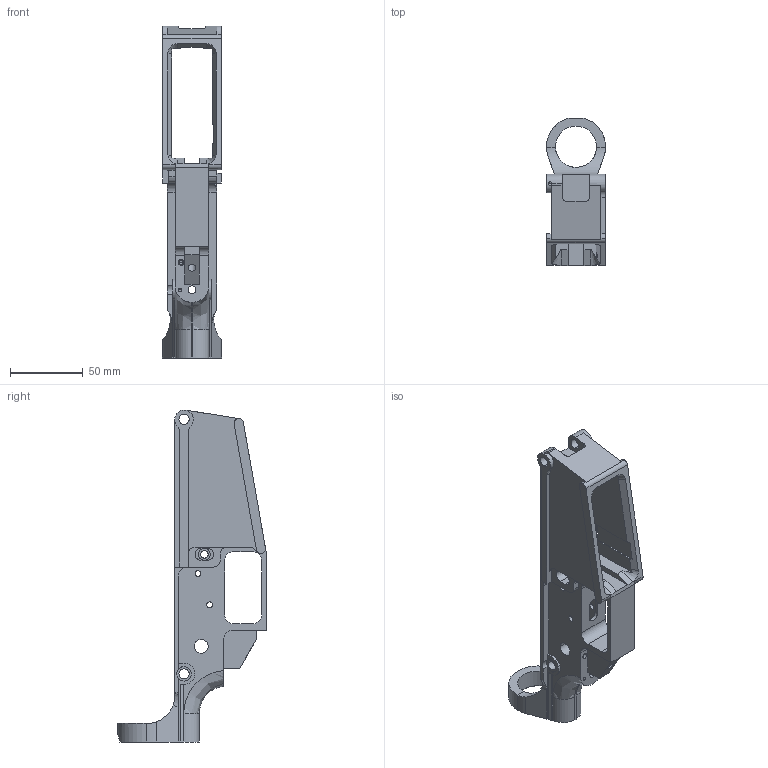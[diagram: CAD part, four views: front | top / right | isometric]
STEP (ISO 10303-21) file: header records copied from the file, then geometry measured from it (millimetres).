
FILE_DESCRIPTION (( 'STEP AP214' ), '1' );
FILE_NAME ('LR308 LOWER.STEP', '2016-04-23T05:09:30', ( '' ), ( '' ), 'SwSTEP 2.0', 'SolidWorks 2013', '' );
FILE_SCHEMA (( 'AUTOMOTIVE_DESIGN' ));
Length unit declared in the file: inch
Products named in the file (1): LR308 LOWER
Bounding box: 40.51 x 101.6 x 227.84 mm (x, y, z)
Volume: 130329.1 mm3; surface area: 63286.4 mm2
Topology: 1 solids, 1 shells, 260 faces, 773 edges, 509 vertices
Faces by surface type: plane 129, cylinder 115, cone 12, bspline 4
Entity records: 9474 total; most frequent: CARTESIAN_POINT 2300, ORIENTED_EDGE 1538, DIRECTION 1466, EDGE_CURVE 769, VERTEX_POINT 509, AXIS2_PLACEMENT_3D 497, VECTOR 472, LINE 472
